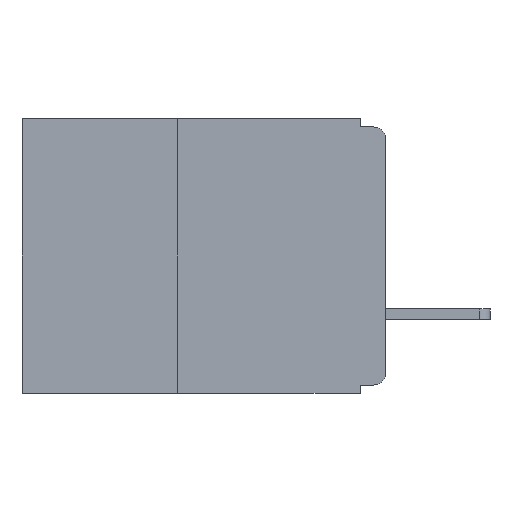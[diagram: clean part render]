
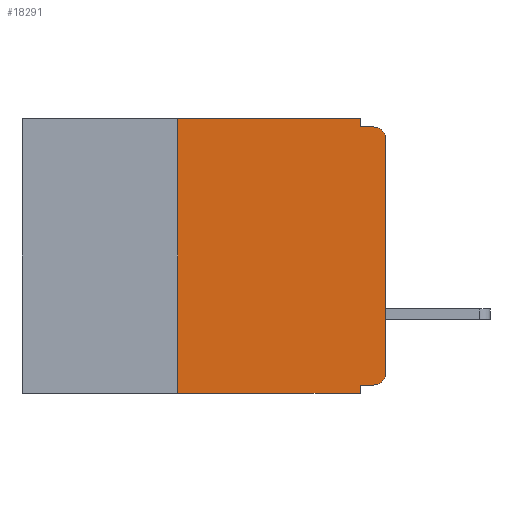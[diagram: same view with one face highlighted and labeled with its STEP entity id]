
A CAD part, left-side view. The second image highlights one B-rep face of the part: STEP entity #18291.
In plain terms, the highlighted planar face has unit normal (-1, 0, 0).
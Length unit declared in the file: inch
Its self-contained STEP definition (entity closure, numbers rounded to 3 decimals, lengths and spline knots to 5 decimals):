
#504 = DIRECTION ( 'NONE',  ( 0., 1., 0. ) ) ;
#656 = CARTESIAN_POINT ( 'NONE',  ( 0., 0.015, -0.32 ) ) ;
#787 = CIRCLE ( 'NONE', #11601, 0.015 ) ;
#839 = CARTESIAN_POINT ( 'NONE',  ( 0., 0., -0.32 ) ) ;
#918 = VECTOR ( 'NONE', #16749, 39.37008 ) ;
#1066 = LINE ( 'NONE', #16938, #918 ) ;
#1121 = VERTEX_POINT ( 'NONE', #14113 ) ;
#1327 = EDGE_LOOP ( 'NONE', ( #9083, #9452, #11095, #13337, #13726, #14407, #16440, #2416, #2941, #3129 ) ) ;
#1461 = DIRECTION ( 'NONE',  ( 0., 0., -1. ) ) ;
#1480 = DIRECTION ( 'NONE',  ( 1., 0., 0. ) ) ;
#1508 = PLANE ( 'NONE',  #16377 ) ;
#2247 = CARTESIAN_POINT ( 'NONE',  ( 0., 0.437, 0. ) ) ;
#2416 = ORIENTED_EDGE ( 'NONE', *, *, #10021, .F. ) ;
#2927 = DIRECTION ( 'NONE',  ( 0., 0., -1. ) ) ;
#2941 = ORIENTED_EDGE ( 'NONE', *, *, #3974, .F. ) ;
#3129 = ORIENTED_EDGE ( 'NONE', *, *, #4969, .T. ) ;
#3563 = EDGE_CURVE ( 'NONE', #3806, #9528, #18153, .T. ) ;
#3806 = VERTEX_POINT ( 'NONE', #15613 ) ;
#3810 = VERTEX_POINT ( 'NONE', #13835 ) ;
#3908 = CARTESIAN_POINT ( 'NONE',  ( 0., 0., -0.025 ) ) ;
#3974 = EDGE_CURVE ( 'NONE', #16491, #3810, #9148, .T. ) ;
#4186 = CARTESIAN_POINT ( 'NONE',  ( 0., 0.031, 0. ) ) ;
#4472 = CARTESIAN_POINT ( 'NONE',  ( 0., 0., 0. ) ) ;
#4969 = EDGE_CURVE ( 'NONE', #16491, #3806, #13405, .T. ) ;
#5352 = EDGE_CURVE ( 'NONE', #18026, #1121, #11908, .T. ) ;
#6050 = VERTEX_POINT ( 'NONE', #11863 ) ;
#6123 = VECTOR ( 'NONE', #18782, 39.37008 ) ;
#6141 = LINE ( 'NONE', #19176, #6123 ) ;
#6195 = DIRECTION ( 'NONE',  ( -1., 0., 0. ) ) ;
#6223 = DIRECTION ( 'NONE',  ( 0., 0., -1. ) ) ;
#6241 = CARTESIAN_POINT ( 'NONE',  ( 0., 0.015, -0.025 ) ) ;
#6551 = AXIS2_PLACEMENT_3D ( 'NONE', #8763, #8666, #8648 ) ;
#6743 = EDGE_CURVE ( 'NONE', #6050, #9690, #6141, .T. ) ;
#7997 = DIRECTION ( 'NONE',  ( 0., 0., 1. ) ) ;
#8237 = CARTESIAN_POINT ( 'NONE',  ( 0., 0.25, -0.33 ) ) ;
#8648 = DIRECTION ( 'NONE',  ( 0., 0., -1. ) ) ;
#8666 = DIRECTION ( 'NONE',  ( -1., 0., 0. ) ) ;
#8763 = CARTESIAN_POINT ( 'NONE',  ( 0., 0.015, -0.305 ) ) ;
#8847 = DIRECTION ( 'NONE',  ( 0., -1., 0. ) ) ;
#9083 = ORIENTED_EDGE ( 'NONE', *, *, #3563, .T. ) ;
#9148 = LINE ( 'NONE', #839, #9466 ) ;
#9371 = DIRECTION ( 'NONE',  ( 0., 0., -1. ) ) ;
#9452 = ORIENTED_EDGE ( 'NONE', *, *, #18046, .T. ) ;
#9466 = VECTOR ( 'NONE', #504, 39.37008 ) ;
#9528 = VERTEX_POINT ( 'NONE', #3908 ) ;
#9568 = CARTESIAN_POINT ( 'NONE',  ( 0., 0.031, -0.33 ) ) ;
#9690 = VERTEX_POINT ( 'NONE', #17680 ) ;
#10021 = EDGE_CURVE ( 'NONE', #3810, #1121, #11463, .T. ) ;
#10077 = CARTESIAN_POINT ( 'NONE',  ( 0., 0.437, -0.33 ) ) ;
#10091 = CARTESIAN_POINT ( 'NONE',  ( 0., 0.031, -0.01 ) ) ;
#11095 = ORIENTED_EDGE ( 'NONE', *, *, #15296, .F. ) ;
#11463 = LINE ( 'NONE', #9568, #11762 ) ;
#11496 = CARTESIAN_POINT ( 'NONE',  ( 0., 0.015, -0.01 ) ) ;
#11601 = AXIS2_PLACEMENT_3D ( 'NONE', #6241, #6195, #6223 ) ;
#11762 = VECTOR ( 'NONE', #9371, 39.37008 ) ;
#11863 = CARTESIAN_POINT ( 'NONE',  ( 0., 0.25, 0. ) ) ;
#11867 = VECTOR ( 'NONE', #8847, 39.37008 ) ;
#11908 = LINE ( 'NONE', #10077, #11867 ) ;
#12348 = EDGE_CURVE ( 'NONE', #18026, #6050, #16100, .T. ) ;
#12494 = CARTESIAN_POINT ( 'NONE',  ( 0., 0.25, -0.33 ) ) ;
#12546 = VERTEX_POINT ( 'NONE', #11496 ) ;
#13337 = ORIENTED_EDGE ( 'NONE', *, *, #16475, .F. ) ;
#13405 = CIRCLE ( 'NONE', #6551, 0.015 ) ;
#13726 = ORIENTED_EDGE ( 'NONE', *, *, #6743, .F. ) ;
#13835 = CARTESIAN_POINT ( 'NONE',  ( 0., 0.031, -0.32 ) ) ;
#14113 = CARTESIAN_POINT ( 'NONE',  ( 0., 0.031, -0.33 ) ) ;
#14407 = ORIENTED_EDGE ( 'NONE', *, *, #12348, .F. ) ;
#14803 = VERTEX_POINT ( 'NONE', #10091 ) ;
#14814 = VECTOR ( 'NONE', #2927, 39.37008 ) ;
#14899 = LINE ( 'NONE', #4186, #14814 ) ;
#15296 = EDGE_CURVE ( 'NONE', #14803, #12546, #1066, .T. ) ;
#15613 = CARTESIAN_POINT ( 'NONE',  ( 0., 0., -0.305 ) ) ;
#16022 = FACE_OUTER_BOUND ( 'NONE', #1327, .T. ) ;
#16083 = VECTOR ( 'NONE', #7997, 39.37008 ) ;
#16100 = LINE ( 'NONE', #8237, #16083 ) ;
#16377 = AXIS2_PLACEMENT_3D ( 'NONE', #2247, #1480, #1461 ) ;
#16440 = ORIENTED_EDGE ( 'NONE', *, *, #5352, .T. ) ;
#16475 = EDGE_CURVE ( 'NONE', #9690, #14803, #14899, .T. ) ;
#16491 = VERTEX_POINT ( 'NONE', #656 ) ;
#16749 = DIRECTION ( 'NONE',  ( 0., -1., 0. ) ) ;
#16938 = CARTESIAN_POINT ( 'NONE',  ( 0., 0., -0.01 ) ) ;
#17374 = VECTOR ( 'NONE', #18608, 39.37008 ) ;
#17680 = CARTESIAN_POINT ( 'NONE',  ( 0., 0.031, 0. ) ) ;
#18026 = VERTEX_POINT ( 'NONE', #12494 ) ;
#18046 = EDGE_CURVE ( 'NONE', #9528, #12546, #787, .T. ) ;
#18153 = LINE ( 'NONE', #4472, #17374 ) ;
#18291 = ADVANCED_FACE ( 'NONE', ( #16022 ), #1508, .F. ) ;
#18608 = DIRECTION ( 'NONE',  ( 0., 0., 1. ) ) ;
#18782 = DIRECTION ( 'NONE',  ( 0., -1., 0. ) ) ;
#19176 = CARTESIAN_POINT ( 'NONE',  ( 0., 0.437, 0. ) ) ;
